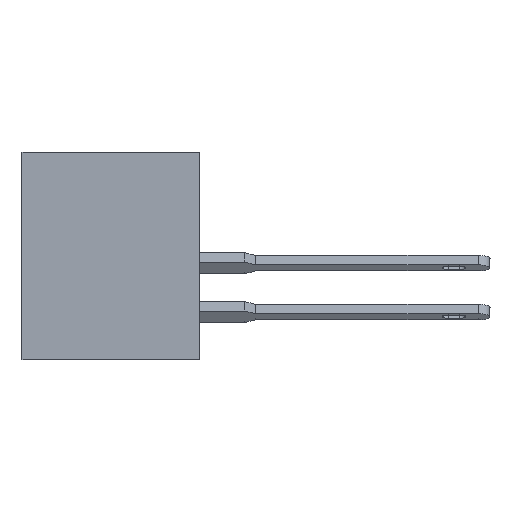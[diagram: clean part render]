
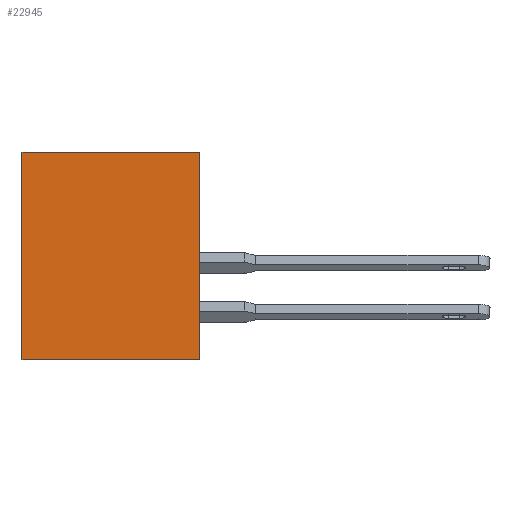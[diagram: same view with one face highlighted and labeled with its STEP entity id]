
A CAD part, left-side view. The second image highlights one B-rep face of the part: STEP entity #22945.
In plain terms, the highlighted planar face has unit normal (-1, 0, 0).
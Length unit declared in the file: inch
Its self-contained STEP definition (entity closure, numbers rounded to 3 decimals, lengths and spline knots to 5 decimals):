
#164 = LINE ( 'NONE', #13129, #7471 ) ;
#1201 = EDGE_CURVE ( 'NONE', #20958, #20649, #4920, .T. ) ;
#2114 = VECTOR ( 'NONE', #4837, 39.37008 ) ;
#2900 = EDGE_CURVE ( 'NONE', #20958, #3455, #20739, .T. ) ;
#3455 = VERTEX_POINT ( 'NONE', #6877 ) ;
#3486 = PLANE ( 'NONE',  #10398 ) ;
#4774 = VERTEX_POINT ( 'NONE', #18161 ) ;
#4837 = DIRECTION ( 'NONE',  ( 0., 0., 1. ) ) ;
#4920 = LINE ( 'NONE', #21843, #11873 ) ;
#5300 = ORIENTED_EDGE ( 'NONE', *, *, #1201, .F. ) ;
#6877 = CARTESIAN_POINT ( 'NONE',  ( 0., 0., -0.531 ) ) ;
#7471 = VECTOR ( 'NONE', #14923, 39.37008 ) ;
#8480 = DIRECTION ( 'NONE',  ( 1., 0., 0. ) ) ;
#9880 = CARTESIAN_POINT ( 'NONE',  ( 0., 0.453, 0. ) ) ;
#10017 = EDGE_CURVE ( 'NONE', #3455, #4774, #16344, .T. ) ;
#10398 = AXIS2_PLACEMENT_3D ( 'NONE', #17675, #8480, #22895 ) ;
#11248 = DIRECTION ( 'NONE',  ( 0., 0., 1. ) ) ;
#11546 = ORIENTED_EDGE ( 'NONE', *, *, #12808, .F. ) ;
#11873 = VECTOR ( 'NONE', #11248, 39.37008 ) ;
#12808 = EDGE_CURVE ( 'NONE', #20649, #4774, #164, .T. ) ;
#13129 = CARTESIAN_POINT ( 'NONE',  ( 0., 0.453, 0. ) ) ;
#14923 = DIRECTION ( 'NONE',  ( 0., -1., 0. ) ) ;
#15907 = FACE_OUTER_BOUND ( 'NONE', #22831, .T. ) ;
#16009 = VECTOR ( 'NONE', #19448, 39.37008 ) ;
#16088 = CARTESIAN_POINT ( 'NONE',  ( 0., 0.453, -0.531 ) ) ;
#16344 = LINE ( 'NONE', #17462, #2114 ) ;
#17462 = CARTESIAN_POINT ( 'NONE',  ( 0., 0., 0. ) ) ;
#17675 = CARTESIAN_POINT ( 'NONE',  ( 0., 0.453, 0. ) ) ;
#18161 = CARTESIAN_POINT ( 'NONE',  ( 0., 0., 0. ) ) ;
#19448 = DIRECTION ( 'NONE',  ( 0., -1., 0. ) ) ;
#20158 = ORIENTED_EDGE ( 'NONE', *, *, #2900, .T. ) ;
#20649 = VERTEX_POINT ( 'NONE', #9880 ) ;
#20739 = LINE ( 'NONE', #16088, #16009 ) ;
#20958 = VERTEX_POINT ( 'NONE', #21559 ) ;
#21559 = CARTESIAN_POINT ( 'NONE',  ( 0., 0.453, -0.531 ) ) ;
#21843 = CARTESIAN_POINT ( 'NONE',  ( 0., 0.453, 0. ) ) ;
#22365 = ORIENTED_EDGE ( 'NONE', *, *, #10017, .T. ) ;
#22831 = EDGE_LOOP ( 'NONE', ( #22365, #11546, #5300, #20158 ) ) ;
#22895 = DIRECTION ( 'NONE',  ( 0., 0., -1. ) ) ;
#22945 = ADVANCED_FACE ( 'NONE', ( #15907 ), #3486, .F. ) ;
